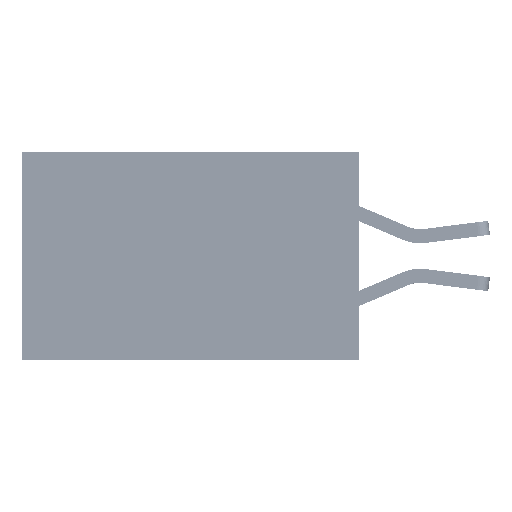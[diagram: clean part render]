
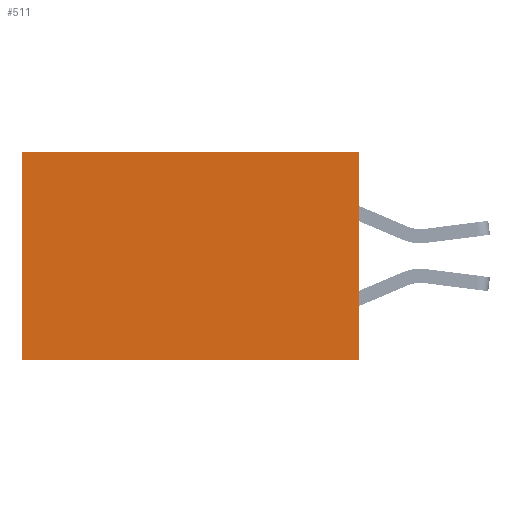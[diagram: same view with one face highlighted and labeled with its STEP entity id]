
A CAD part, left-side view. The second image highlights one B-rep face of the part: STEP entity #511.
In plain terms, the highlighted planar face has unit normal (-1, 0, 0).
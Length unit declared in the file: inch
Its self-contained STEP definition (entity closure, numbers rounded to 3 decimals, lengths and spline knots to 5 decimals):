
#511 = ADVANCED_FACE ( 'NONE', ( #24298 ), #7489, .F. ) ;
#698 = ORIENTED_EDGE ( 'NONE', *, *, #30279, .T. ) ;
#1040 = EDGE_LOOP ( 'NONE', ( #698, #4972, #9014, #3352 ) ) ;
#1057 = EDGE_CURVE ( 'NONE', #10698, #28501, #8830, .T. ) ;
#1600 = DIRECTION ( 'NONE',  ( 0., 1., 0. ) ) ;
#2058 = CARTESIAN_POINT ( 'NONE',  ( 0.2875, 0., -0.37 ) ) ;
#2957 = DIRECTION ( 'NONE',  ( 0., 0., -1. ) ) ;
#3352 = ORIENTED_EDGE ( 'NONE', *, *, #30197, .T. ) ;
#4622 = DIRECTION ( 'NONE',  ( 1., 0., 0. ) ) ;
#4972 = ORIENTED_EDGE ( 'NONE', *, *, #32806, .F. ) ;
#5294 = LINE ( 'NONE', #15406, #8756 ) ;
#7222 = DIRECTION ( 'NONE',  ( 0., 0., -1. ) ) ;
#7489 = PLANE ( 'NONE',  #8922 ) ;
#8651 = CARTESIAN_POINT ( 'NONE',  ( 0.2875, 0., 0. ) ) ;
#8756 = VECTOR ( 'NONE', #7222, 39.37008 ) ;
#8830 = LINE ( 'NONE', #30458, #25156 ) ;
#8922 = AXIS2_PLACEMENT_3D ( 'NONE', #32255, #4622, #26340 ) ;
#9014 = ORIENTED_EDGE ( 'NONE', *, *, #1057, .F. ) ;
#10698 = VERTEX_POINT ( 'NONE', #8651 ) ;
#11489 = CARTESIAN_POINT ( 'NONE',  ( 0.2875, 0.6, 0. ) ) ;
#13840 = CARTESIAN_POINT ( 'NONE',  ( 0.2875, 0., -0.37 ) ) ;
#15406 = CARTESIAN_POINT ( 'NONE',  ( 0.2875, 0.6, 0. ) ) ;
#15540 = CARTESIAN_POINT ( 'NONE',  ( 0.2875, 0.6, -0.37 ) ) ;
#16100 = VECTOR ( 'NONE', #1600, 39.37008 ) ;
#18935 = VECTOR ( 'NONE', #23407, 39.37008 ) ;
#21298 = VERTEX_POINT ( 'NONE', #15540 ) ;
#23407 = DIRECTION ( 'NONE',  ( 0., 1., 0. ) ) ;
#23648 = CARTESIAN_POINT ( 'NONE',  ( 0.2875, 0., 0. ) ) ;
#24298 = FACE_OUTER_BOUND ( 'NONE', #1040, .T. ) ;
#25156 = VECTOR ( 'NONE', #2957, 39.37008 ) ;
#26340 = DIRECTION ( 'NONE',  ( 0., 0., -1. ) ) ;
#28501 = VERTEX_POINT ( 'NONE', #13840 ) ;
#30197 = EDGE_CURVE ( 'NONE', #10698, #35056, #33678, .T. ) ;
#30279 = EDGE_CURVE ( 'NONE', #35056, #21298, #5294, .T. ) ;
#30458 = CARTESIAN_POINT ( 'NONE',  ( 0.2875, 0., 0. ) ) ;
#32255 = CARTESIAN_POINT ( 'NONE',  ( 0.2875, 0., 0. ) ) ;
#32806 = EDGE_CURVE ( 'NONE', #28501, #21298, #33596, .T. ) ;
#33596 = LINE ( 'NONE', #2058, #18935 ) ;
#33678 = LINE ( 'NONE', #23648, #16100 ) ;
#35056 = VERTEX_POINT ( 'NONE', #11489 ) ;
